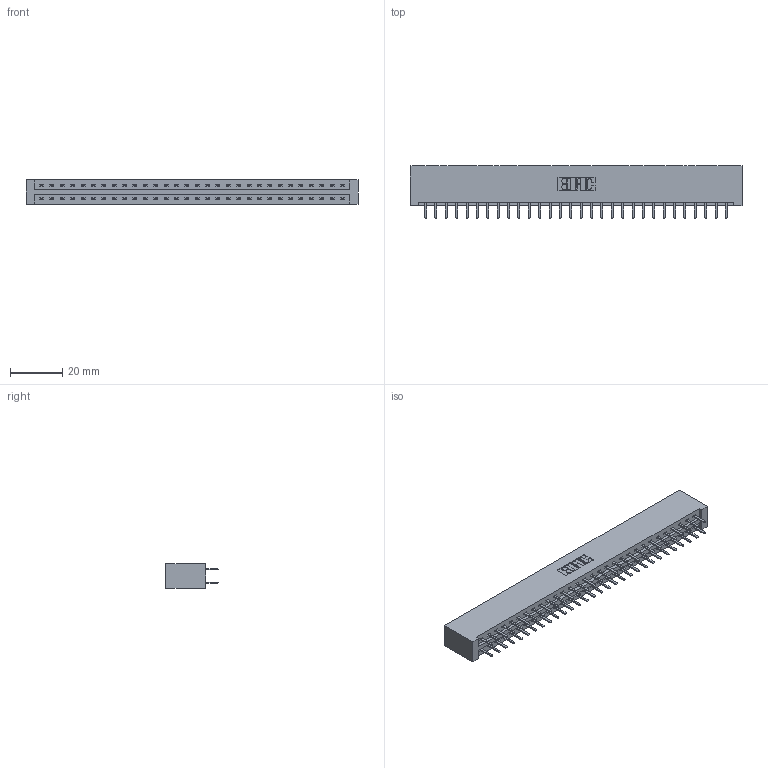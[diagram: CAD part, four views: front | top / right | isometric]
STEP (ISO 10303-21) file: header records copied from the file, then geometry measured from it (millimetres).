
FILE_DESCRIPTION (( 'STEP AP203' ), '1' );
FILE_NAME ('387-060-520-201.STEP', '2018-09-21T02:35:56', ( '' ), ( '' ), 'SwSTEP 2.0', 'SolidWorks 2016', '' );
FILE_SCHEMA (( 'CONFIG_CONTROL_DESIGN' ));
Length unit declared in the file: inch
Products named in the file (3): 337 Part_No Mounting Lugs; 345-292-001_345-293-120; 387-060-520-201
Assembly tree (61 placements, depth 2):
  387-060-520-201
    337 Part_No Mounting Lugs
    345-292-001_345-293-120  x60
Bounding box: 126.75 x 20.02 x 9.4 mm (x, y, z)
Volume: 13932.1 mm3; surface area: 15614.6 mm2
Topology: 61 solids, 61 shells, 3586 faces, 10427 edges, 6790 vertices
Faces by surface type: plane 2466, cylinder 1120
Entity records: 24649 total; most frequent: CARTESIAN_POINT 4174, ORIENTED_EDGE 4098, DIRECTION 3553, EDGE_CURVE 2049, VECTOR 1925, LINE 1925, VERTEX_POINT 1362, AXIS2_PLACEMENT_3D 814
